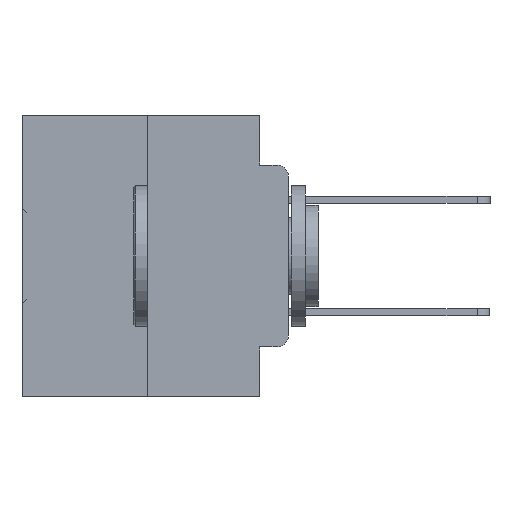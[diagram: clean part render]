
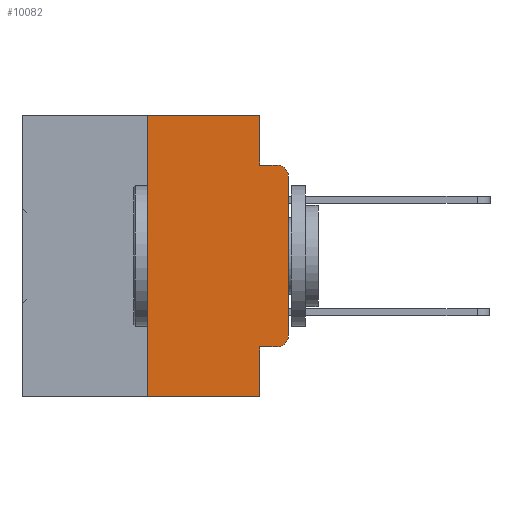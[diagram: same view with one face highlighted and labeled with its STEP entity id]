
A CAD part, left-side view. The second image highlights one B-rep face of the part: STEP entity #10082.
In plain terms, the highlighted planar face has unit normal (-1, 0, 0).
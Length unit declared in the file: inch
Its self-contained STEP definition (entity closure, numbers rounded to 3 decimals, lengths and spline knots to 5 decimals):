
#688 = DIRECTION ( 'NONE',  ( -1., 0., 0. ) ) ;
#1128 = VERTEX_POINT ( 'NONE', #19815 ) ;
#1564 = LINE ( 'NONE', #25534, #2431 ) ;
#1663 = ORIENTED_EDGE ( 'NONE', *, *, #21899, .F. ) ;
#1710 = CIRCLE ( 'NONE', #21796, 0.02 ) ;
#2431 = VECTOR ( 'NONE', #27493, 39.37008 ) ;
#2522 = CARTESIAN_POINT ( 'NONE',  ( 0., 0.25, -0.5 ) ) ;
#3074 = VECTOR ( 'NONE', #8317, 39.37008 ) ;
#3448 = VECTOR ( 'NONE', #20683, 39.37008 ) ;
#3711 = CARTESIAN_POINT ( 'NONE',  ( 0., 0.02, -0.0885 ) ) ;
#4431 = CARTESIAN_POINT ( 'NONE',  ( 0., 0.051, 0. ) ) ;
#5435 = VECTOR ( 'NONE', #31860, 39.37008 ) ;
#6161 = LINE ( 'NONE', #19493, #12587 ) ;
#6602 = EDGE_CURVE ( 'NONE', #18212, #23525, #1710, .T. ) ;
#6757 = CIRCLE ( 'NONE', #28754, 0.02 ) ;
#7157 = DIRECTION ( 'NONE',  ( 0., 0., -1. ) ) ;
#7262 = DIRECTION ( 'NONE',  ( 1., 0., 0. ) ) ;
#7290 = ORIENTED_EDGE ( 'NONE', *, *, #22579, .F. ) ;
#7909 = CARTESIAN_POINT ( 'NONE',  ( 0., 0.051, 0. ) ) ;
#8253 = EDGE_CURVE ( 'NONE', #1128, #35469, #6757, .T. ) ;
#8317 = DIRECTION ( 'NONE',  ( 0., 0., 1. ) ) ;
#8411 = LINE ( 'NONE', #4431, #35097 ) ;
#8560 = FACE_OUTER_BOUND ( 'NONE', #24622, .T. ) ;
#9023 = LINE ( 'NONE', #15060, #3448 ) ;
#10082 = ADVANCED_FACE ( 'NONE', ( #8560 ), #18272, .F. ) ;
#10730 = ORIENTED_EDGE ( 'NONE', *, *, #15816, .T. ) ;
#11215 = LINE ( 'NONE', #22090, #3074 ) ;
#11658 = AXIS2_PLACEMENT_3D ( 'NONE', #31993, #7262, #26599 ) ;
#12587 = VECTOR ( 'NONE', #22275, 39.37008 ) ;
#12767 = CARTESIAN_POINT ( 'NONE',  ( 0., 0.051, 0. ) ) ;
#13203 = VERTEX_POINT ( 'NONE', #25853 ) ;
#14040 = CARTESIAN_POINT ( 'NONE',  ( 0., 0., -0.3915 ) ) ;
#14288 = EDGE_CURVE ( 'NONE', #19044, #13203, #6161, .T. ) ;
#14367 = VECTOR ( 'NONE', #32094, 39.37008 ) ;
#14538 = VERTEX_POINT ( 'NONE', #23333 ) ;
#15023 = ORIENTED_EDGE ( 'NONE', *, *, #31797, .F. ) ;
#15060 = CARTESIAN_POINT ( 'NONE',  ( 0., 0.051, -0.4115 ) ) ;
#15223 = CARTESIAN_POINT ( 'NONE',  ( 0., 0.02, -0.3915 ) ) ;
#15302 = CARTESIAN_POINT ( 'NONE',  ( 0., 0.473, 0. ) ) ;
#15816 = EDGE_CURVE ( 'NONE', #32881, #18212, #9023, .T. ) ;
#16990 = CARTESIAN_POINT ( 'NONE',  ( 0., 0.051, -0.4115 ) ) ;
#17219 = CARTESIAN_POINT ( 'NONE',  ( 0., 0.02, -0.1085 ) ) ;
#17822 = EDGE_CURVE ( 'NONE', #24813, #31240, #33885, .T. ) ;
#18061 = DIRECTION ( 'NONE',  ( 0., 0., -1. ) ) ;
#18212 = VERTEX_POINT ( 'NONE', #22567 ) ;
#18272 = PLANE ( 'NONE',  #11658 ) ;
#19044 = VERTEX_POINT ( 'NONE', #2522 ) ;
#19493 = CARTESIAN_POINT ( 'NONE',  ( 0., 0.473, -0.5 ) ) ;
#19815 = CARTESIAN_POINT ( 'NONE',  ( 0., 0., -0.1085 ) ) ;
#19871 = ORIENTED_EDGE ( 'NONE', *, *, #6602, .T. ) ;
#20014 = DIRECTION ( 'NONE',  ( 0., 0., -1. ) ) ;
#20256 = ORIENTED_EDGE ( 'NONE', *, *, #8253, .T. ) ;
#20683 = DIRECTION ( 'NONE',  ( 0., -1., 0. ) ) ;
#20706 = ORIENTED_EDGE ( 'NONE', *, *, #17822, .F. ) ;
#21759 = LINE ( 'NONE', #12767, #14367 ) ;
#21796 = AXIS2_PLACEMENT_3D ( 'NONE', #15223, #34511, #18061 ) ;
#21899 = EDGE_CURVE ( 'NONE', #31240, #14538, #8411, .T. ) ;
#21975 = ORIENTED_EDGE ( 'NONE', *, *, #27438, .F. ) ;
#22090 = CARTESIAN_POINT ( 'NONE',  ( 0., 0., 0. ) ) ;
#22275 = DIRECTION ( 'NONE',  ( 0., -1., 0. ) ) ;
#22567 = CARTESIAN_POINT ( 'NONE',  ( 0., 0.02, -0.4115 ) ) ;
#22579 = EDGE_CURVE ( 'NONE', #32881, #13203, #21759, .T. ) ;
#23333 = CARTESIAN_POINT ( 'NONE',  ( 0., 0.051, -0.0885 ) ) ;
#23525 = VERTEX_POINT ( 'NONE', #14040 ) ;
#23627 = LINE ( 'NONE', #35186, #30961 ) ;
#24622 = EDGE_LOOP ( 'NONE', ( #30569, #20256, #21975, #1663, #20706, #15023, #29740, #7290, #10730, #19871 ) ) ;
#24813 = VERTEX_POINT ( 'NONE', #29905 ) ;
#24930 = EDGE_CURVE ( 'NONE', #23525, #1128, #11215, .T. ) ;
#25534 = CARTESIAN_POINT ( 'NONE',  ( 0., 0.051, -0.0885 ) ) ;
#25853 = CARTESIAN_POINT ( 'NONE',  ( 0., 0.051, -0.5 ) ) ;
#26599 = DIRECTION ( 'NONE',  ( 0., 0., -1. ) ) ;
#27064 = DIRECTION ( 'NONE',  ( 0., 0., 1. ) ) ;
#27438 = EDGE_CURVE ( 'NONE', #14538, #35469, #1564, .T. ) ;
#27493 = DIRECTION ( 'NONE',  ( 0., -1., 0. ) ) ;
#28754 = AXIS2_PLACEMENT_3D ( 'NONE', #17219, #688, #20014 ) ;
#29740 = ORIENTED_EDGE ( 'NONE', *, *, #14288, .T. ) ;
#29905 = CARTESIAN_POINT ( 'NONE',  ( 0., 0.25, 0. ) ) ;
#30569 = ORIENTED_EDGE ( 'NONE', *, *, #24930, .T. ) ;
#30961 = VECTOR ( 'NONE', #27064, 39.37008 ) ;
#31240 = VERTEX_POINT ( 'NONE', #7909 ) ;
#31797 = EDGE_CURVE ( 'NONE', #19044, #24813, #23627, .T. ) ;
#31860 = DIRECTION ( 'NONE',  ( 0., -1., 0. ) ) ;
#31993 = CARTESIAN_POINT ( 'NONE',  ( 0., 0.473, 0. ) ) ;
#32094 = DIRECTION ( 'NONE',  ( 0., 0., -1. ) ) ;
#32881 = VERTEX_POINT ( 'NONE', #16990 ) ;
#33885 = LINE ( 'NONE', #15302, #5435 ) ;
#34511 = DIRECTION ( 'NONE',  ( -1., 0., 0. ) ) ;
#35097 = VECTOR ( 'NONE', #7157, 39.37008 ) ;
#35186 = CARTESIAN_POINT ( 'NONE',  ( 0., 0.25, 0. ) ) ;
#35469 = VERTEX_POINT ( 'NONE', #3711 ) ;
